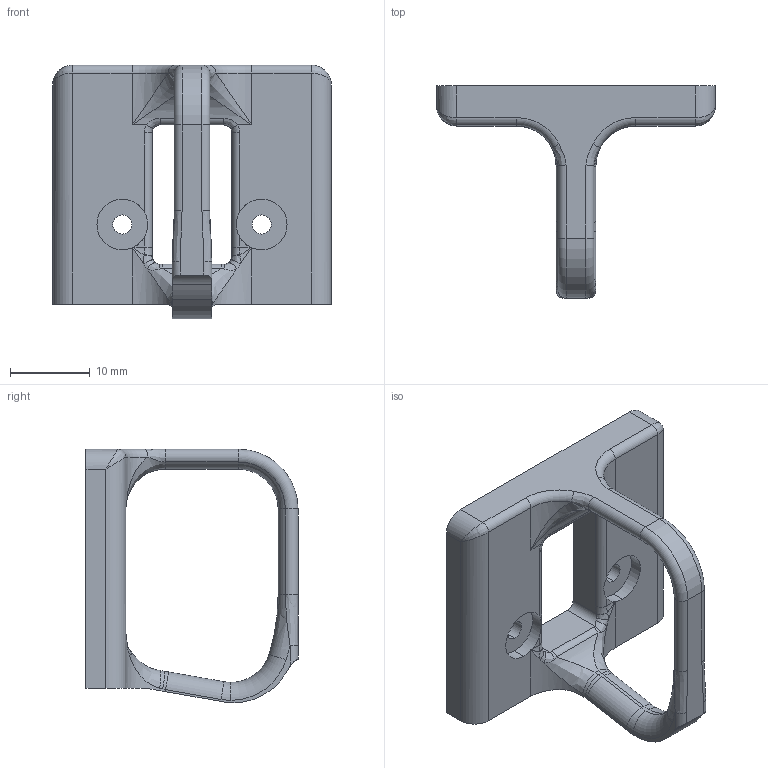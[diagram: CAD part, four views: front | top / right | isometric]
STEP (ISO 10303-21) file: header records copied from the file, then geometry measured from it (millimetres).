
FILE_DESCRIPTION (( 'STEP AP203' ), '1' );
FILE_NAME ('Trigger_Guard.STEP', '2013-11-10T07:44:58', ( '' ), ( '' ), 'SwSTEP 2.0', 'SolidWorks 2013', '' );
FILE_SCHEMA (( 'CONFIG_CONTROL_DESIGN' ));
Length unit declared in the file: millimetre
Products named in the file (1): Trigger_Guard
Bounding box: 35 x 26.63 x 31.84 mm (x, y, z)
Volume: 4952 mm3; surface area: 3438.9 mm2
Topology: 1 solids, 1 shells, 118 faces, 293 edges, 168 vertices
Faces by surface type: cylinder 50, bspline 28, plane 24, torus 16
Entity records: 4178 total; most frequent: CARTESIAN_POINT 1502, ORIENTED_EDGE 574, DIRECTION 531, EDGE_CURVE 287, AXIS2_PLACEMENT_3D 215, VERTEX_POINT 168, CIRCLE 124, EDGE_LOOP 123
